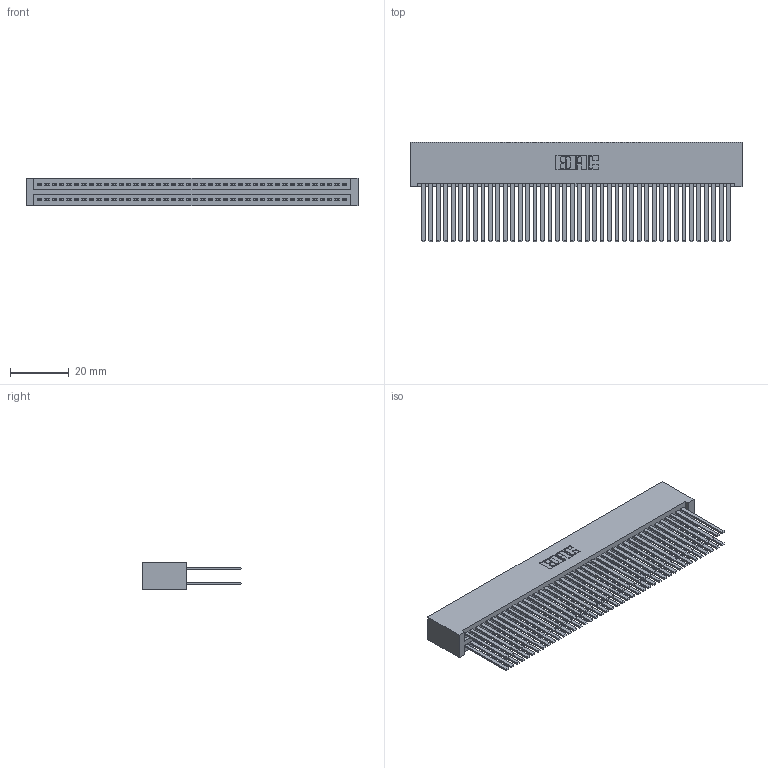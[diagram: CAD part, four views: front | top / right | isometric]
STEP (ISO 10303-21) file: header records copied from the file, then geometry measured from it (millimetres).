
FILE_DESCRIPTION (( 'STEP AP203' ), '1' );
FILE_NAME ('395-084-544-201.STEP', '2018-11-28T14:56:54', ( '' ), ( '' ), 'SwSTEP 2.0', 'SolidWorks 2016', '' );
FILE_SCHEMA (( 'CONFIG_CONTROL_DESIGN' ));
Length unit declared in the file: inch
Products named in the file (3): 345 Part_No Mounting Lugs; 395-084-544-201; 345-292-001_345-293-144
Assembly tree (85 placements, depth 2):
  395-084-544-201
    345 Part_No Mounting Lugs
    345-292-001_345-293-144  x84
Bounding box: 113.28 x 33.96 x 9.4 mm (x, y, z)
Volume: 12798 mm3; surface area: 22672 mm2
Topology: 85 solids, 85 shells, 3814 faces, 11321 edges, 7434 vertices
Faces by surface type: plane 2512, cylinder 1302
Entity records: 32493 total; most frequent: CARTESIAN_POINT 5444, ORIENTED_EDGE 5378, DIRECTION 4793, EDGE_CURVE 2689, LINE 2401, VECTOR 2401, VERTEX_POINT 1790, AXIS2_PLACEMENT_3D 1196
